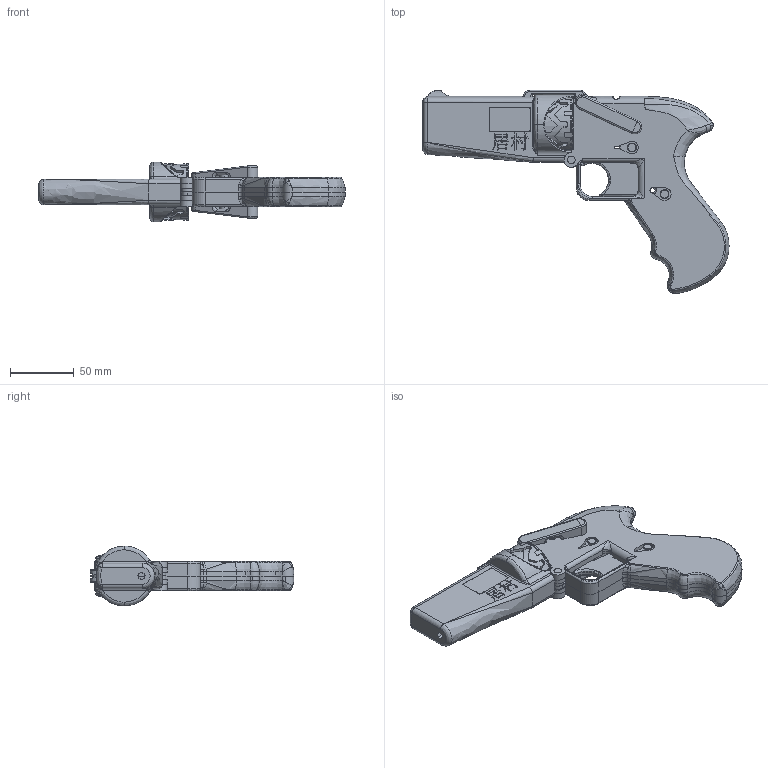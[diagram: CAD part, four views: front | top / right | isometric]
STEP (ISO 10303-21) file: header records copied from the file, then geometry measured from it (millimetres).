
FILE_DESCRIPTION (( 'STEP AP214' ), '1' );
FILE_NAME ('Imura_V2_Complete.step', '2015-01-26T00:09:03', ( 'WarFairy' ), ( '' ), 'SwSTEP 2.0', 'SolidWorks 2013', '' );
FILE_SCHEMA (( 'AUTOMOTIVE_DESIGN' ));
Length unit declared in the file: millimetre
Products named in the file (19): Imura_V2_Trigger; Imura_V2_Complete; Imura_V2_Flapper_Pin; Imura_V2_Barrel_Weight_Cap; Imura_V2_Trigger_Pin; Imura_V2_Striker_Right; Imura_V2_Striker_Left; Imura_V2_Frame_Pins; Imura_V2_Frame_Right; Imura_V2_Cylinder_Cap; Imura_V2_Release_Lever_Right; Imura_V2_Release_Lever_Left; Imura_V2_Forward_Trigger_Bar; Imura_V2_Latch; Imura_V2_Cylinder; Imura_V2_Frame_Left; Imura_V2_Barrel; Imura_V2_Sear_Flapper; Imura_V2_Sear
Assembly tree (19 placements, depth 2):
  Imura_V2_Complete
    Imura_V2_Trigger
    Imura_V2_Sear
    Imura_V2_Sear_Flapper
    Imura_V2_Barrel
    Imura_V2_Frame_Left
    Imura_V2_Cylinder
    Imura_V2_Latch
    Imura_V2_Forward_Trigger_Bar
    Imura_V2_Release_Lever_Left
    Imura_V2_Release_Lever_Right
    Imura_V2_Cylinder_Cap
    Imura_V2_Frame_Right
    Imura_V2_Frame_Pins  x2
    Imura_V2_Striker_Left
    Imura_V2_Striker_Right
    Imura_V2_Trigger_Pin
    Imura_V2_Barrel_Weight_Cap
    Imura_V2_Flapper_Pin
Bounding box: 239.93 x 159.32 x 47 mm (x, y, z)
Volume: 212311.5 mm3; surface area: 127010.2 mm2
Topology: 18 solids, 19 shells, 1774 faces, 4697 edges, 2951 vertices
Faces by surface type: plane 619, bspline 565, cylinder 560, cone 29, torus 1
Entity records: 102381 total; most frequent: CARTESIAN_POINT 61919, ORIENTED_EDGE 9254, DIRECTION 7002, EDGE_CURVE 4628, VERTEX_POINT 2947, AXIS2_PLACEMENT_3D 2440, LINE 2122, VECTOR 2122
